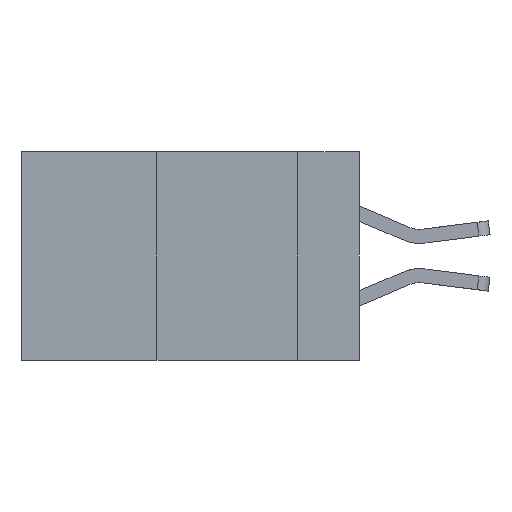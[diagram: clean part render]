
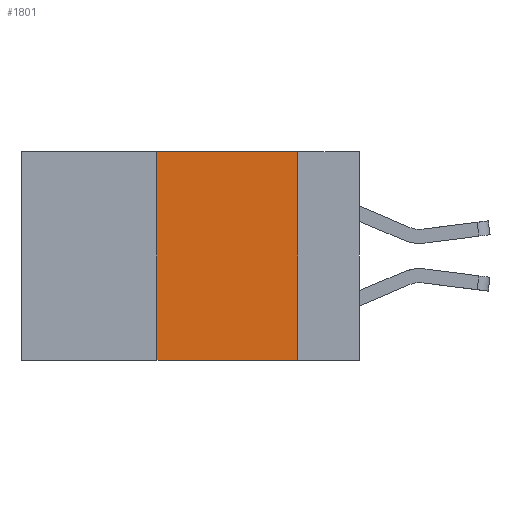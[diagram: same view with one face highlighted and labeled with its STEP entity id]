
A CAD part, left-side view. The second image highlights one B-rep face of the part: STEP entity #1801.
In plain terms, the highlighted planar face has unit normal (-1, 0, 0).
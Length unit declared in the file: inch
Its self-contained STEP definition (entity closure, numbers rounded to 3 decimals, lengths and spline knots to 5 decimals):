
#45 = LINE ( 'NONE', #7066, #5512 ) ;
#358 = LINE ( 'NONE', #13757, #8675 ) ;
#864 = LINE ( 'NONE', #9507, #9534 ) ;
#1016 = PLANE ( 'NONE',  #4951 ) ;
#1093 = DIRECTION ( 'NONE',  ( 0., 0., -1. ) ) ;
#1096 = DIRECTION ( 'NONE',  ( 1., 0., 0. ) ) ;
#1801 = ADVANCED_FACE ( 'NONE', ( #9322 ), #1016, .F. ) ;
#1890 = CARTESIAN_POINT ( 'NONE',  ( 0., 0.11, 0. ) ) ;
#1920 = DIRECTION ( 'NONE',  ( 0., -1., 0. ) ) ;
#2007 = EDGE_LOOP ( 'NONE', ( #10813, #7837, #12405, #10505 ) ) ;
#2193 = LINE ( 'NONE', #3521, #8282 ) ;
#3186 = VERTEX_POINT ( 'NONE', #8061 ) ;
#3521 = CARTESIAN_POINT ( 'NONE',  ( 0., 0.6, -0.37 ) ) ;
#4859 = VERTEX_POINT ( 'NONE', #1890 ) ;
#4951 = AXIS2_PLACEMENT_3D ( 'NONE', #13140, #1096, #1093 ) ;
#5512 = VECTOR ( 'NONE', #11306, 39.37008 ) ;
#5544 = VERTEX_POINT ( 'NONE', #11431 ) ;
#7066 = CARTESIAN_POINT ( 'NONE',  ( 0., 0.36, 0. ) ) ;
#7287 = EDGE_CURVE ( 'NONE', #4859, #3186, #358, .T. ) ;
#7553 = VERTEX_POINT ( 'NONE', #11298 ) ;
#7746 = EDGE_CURVE ( 'NONE', #7553, #4859, #864, .T. ) ;
#7837 = ORIENTED_EDGE ( 'NONE', *, *, #7746, .F. ) ;
#8061 = CARTESIAN_POINT ( 'NONE',  ( 0., 0.11, -0.37 ) ) ;
#8282 = VECTOR ( 'NONE', #11024, 39.37008 ) ;
#8600 = DIRECTION ( 'NONE',  ( 0., 0., -1. ) ) ;
#8675 = VECTOR ( 'NONE', #8600, 39.37008 ) ;
#9322 = FACE_OUTER_BOUND ( 'NONE', #2007, .T. ) ;
#9507 = CARTESIAN_POINT ( 'NONE',  ( 0., 0.6, 0. ) ) ;
#9534 = VECTOR ( 'NONE', #1920, 39.37008 ) ;
#9730 = EDGE_CURVE ( 'NONE', #5544, #3186, #2193, .T. ) ;
#10505 = ORIENTED_EDGE ( 'NONE', *, *, #9730, .T. ) ;
#10813 = ORIENTED_EDGE ( 'NONE', *, *, #7287, .F. ) ;
#11024 = DIRECTION ( 'NONE',  ( 0., -1., 0. ) ) ;
#11298 = CARTESIAN_POINT ( 'NONE',  ( 0., 0.36, 0. ) ) ;
#11306 = DIRECTION ( 'NONE',  ( 0., 0., 1. ) ) ;
#11431 = CARTESIAN_POINT ( 'NONE',  ( 0., 0.36, -0.37 ) ) ;
#12405 = ORIENTED_EDGE ( 'NONE', *, *, #13822, .F. ) ;
#13140 = CARTESIAN_POINT ( 'NONE',  ( 0., 0.6, 0. ) ) ;
#13757 = CARTESIAN_POINT ( 'NONE',  ( 0., 0.11, 0. ) ) ;
#13822 = EDGE_CURVE ( 'NONE', #5544, #7553, #45, .T. ) ;
